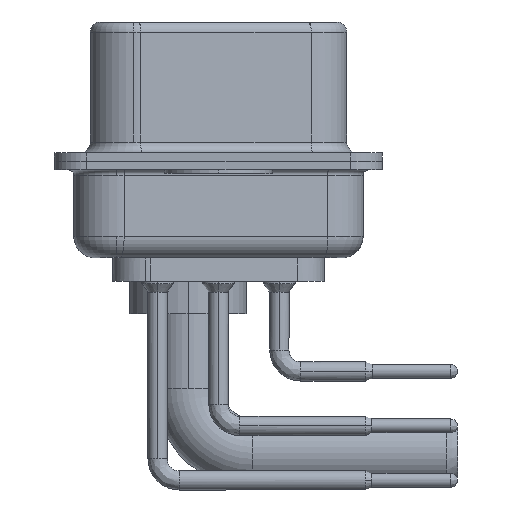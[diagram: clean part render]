
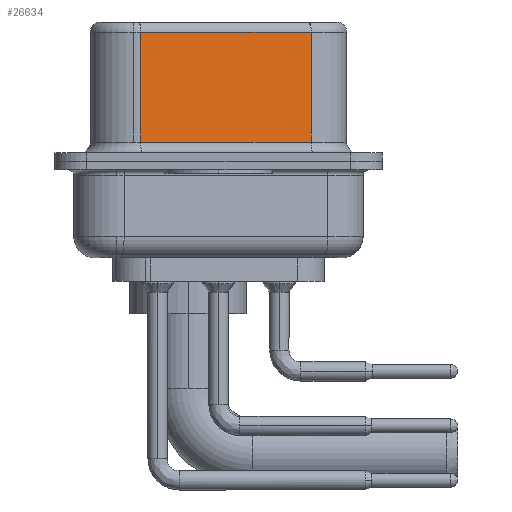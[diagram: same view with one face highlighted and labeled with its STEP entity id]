
A CAD part, left-side view. The second image highlights one B-rep face of the part: STEP entity #26634.
In plain terms, the highlighted planar face has unit normal (-0.985, -0.174, 0).
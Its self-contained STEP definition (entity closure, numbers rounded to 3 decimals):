
#96 = DIRECTION ( 'NONE',  ( 0.985, 0.174, 0. ) ) ;
#213 = VERTEX_POINT ( 'NONE', #2889 ) ;
#444 = DIRECTION ( 'NONE',  ( 0., 0., -1. ) ) ;
#881 = AXIS2_PLACEMENT_3D ( 'NONE', #26725, #96, #23947 ) ;
#1878 = ORIENTED_EDGE ( 'NONE', *, *, #10113, .T. ) ;
#2889 = CARTESIAN_POINT ( 'NONE',  ( 3.73, 3.628, 6.02 ) ) ;
#5036 = CARTESIAN_POINT ( 'NONE',  ( 3.73, 3.628, 6.52 ) ) ;
#7217 = VECTOR ( 'NONE', #33978, 1000. ) ;
#7412 = FACE_OUTER_BOUND ( 'NONE', #7584, .T. ) ;
#7584 = EDGE_LOOP ( 'NONE', ( #19521, #30303, #15543, #1878 ) ) ;
#9343 = EDGE_CURVE ( 'NONE', #20948, #26568, #16286, .T. ) ;
#9485 = VECTOR ( 'NONE', #33418, 1000. ) ;
#10113 = EDGE_CURVE ( 'NONE', #15750, #26568, #17375, .T. ) ;
#10434 = LINE ( 'NONE', #5036, #19174 ) ;
#13700 = CARTESIAN_POINT ( 'NONE',  ( 5.132, -4.322, 6.52 ) ) ;
#15185 = EDGE_CURVE ( 'NONE', #213, #15750, #10434, .T. ) ;
#15543 = ORIENTED_EDGE ( 'NONE', *, *, #15185, .T. ) ;
#15750 = VERTEX_POINT ( 'NONE', #20639 ) ;
#16286 = LINE ( 'NONE', #13700, #30575 ) ;
#17375 = LINE ( 'NONE', #22793, #9485 ) ;
#19174 = VECTOR ( 'NONE', #26113, 1000. ) ;
#19521 = ORIENTED_EDGE ( 'NONE', *, *, #9343, .F. ) ;
#19820 = EDGE_CURVE ( 'NONE', #20948, #213, #20043, .T. ) ;
#20043 = LINE ( 'NONE', #31348, #7217 ) ;
#20639 = CARTESIAN_POINT ( 'NONE',  ( 3.73, 3.628, 0.9 ) ) ;
#20948 = VERTEX_POINT ( 'NONE', #22671 ) ;
#22671 = CARTESIAN_POINT ( 'NONE',  ( 5.132, -4.322, 6.02 ) ) ;
#22793 = CARTESIAN_POINT ( 'NONE',  ( 5.132, -4.322, 0.9 ) ) ;
#23947 = DIRECTION ( 'NONE',  ( -0.174, 0.985, 0. ) ) ;
#26113 = DIRECTION ( 'NONE',  ( 0., 0., -1. ) ) ;
#26568 = VERTEX_POINT ( 'NONE', #34424 ) ;
#26634 = ADVANCED_FACE ( 'NONE', ( #7412 ), #28662, .F. ) ;
#26725 = CARTESIAN_POINT ( 'NONE',  ( 5.132, -4.322, 6.52 ) ) ;
#28662 = PLANE ( 'NONE',  #881 ) ;
#30303 = ORIENTED_EDGE ( 'NONE', *, *, #19820, .T. ) ;
#30575 = VECTOR ( 'NONE', #444, 1000. ) ;
#31348 = CARTESIAN_POINT ( 'NONE',  ( 5.132, -4.322, 6.02 ) ) ;
#33418 = DIRECTION ( 'NONE',  ( 0.174, -0.985, 0. ) ) ;
#33978 = DIRECTION ( 'NONE',  ( -0.174, 0.985, 0. ) ) ;
#34424 = CARTESIAN_POINT ( 'NONE',  ( 5.132, -4.322, 0.9 ) ) ;
